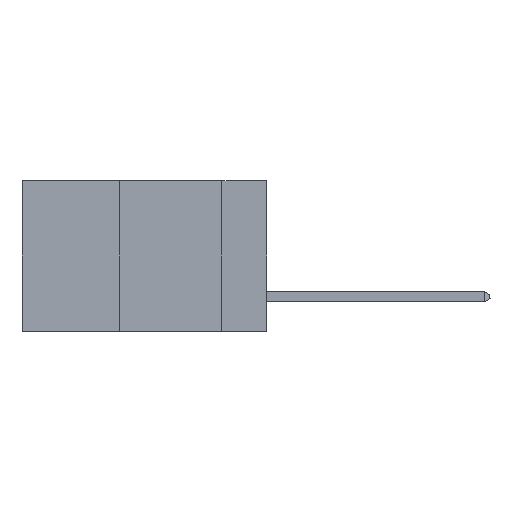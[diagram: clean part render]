
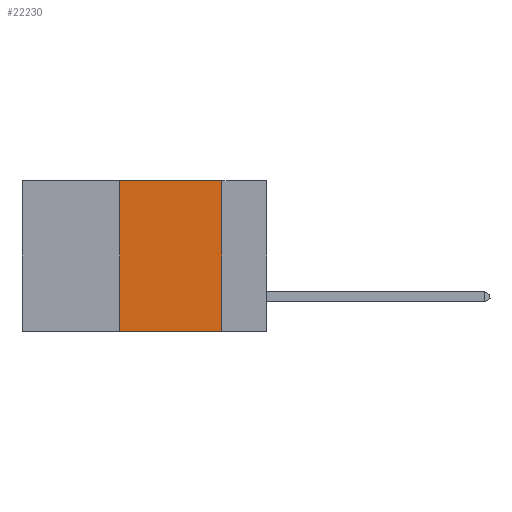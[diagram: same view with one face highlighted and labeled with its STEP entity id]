
A CAD part, left-side view. The second image highlights one B-rep face of the part: STEP entity #22230.
In plain terms, the highlighted planar face has unit normal (-1, 0, 0).
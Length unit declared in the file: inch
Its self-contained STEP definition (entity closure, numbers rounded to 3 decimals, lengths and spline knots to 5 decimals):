
#1137 = FACE_OUTER_BOUND ( 'NONE', #7676, .T. ) ;
#1531 = DIRECTION ( 'NONE',  ( 1., 0., 0. ) ) ;
#2858 = CARTESIAN_POINT ( 'NONE',  ( 0., 0.6, 0. ) ) ;
#3223 = LINE ( 'NONE', #14112, #16207 ) ;
#3950 = EDGE_CURVE ( 'NONE', #8051, #13573, #15029, .T. ) ;
#3980 = CARTESIAN_POINT ( 'NONE',  ( 0., 0.36, -0.37 ) ) ;
#4600 = CARTESIAN_POINT ( 'NONE',  ( 0., 0.36, 0. ) ) ;
#5173 = VERTEX_POINT ( 'NONE', #3980 ) ;
#5322 = PLANE ( 'NONE',  #8281 ) ;
#5871 = DIRECTION ( 'NONE',  ( 0., 0., 1. ) ) ;
#6037 = ORIENTED_EDGE ( 'NONE', *, *, #23399, .F. ) ;
#7606 = VECTOR ( 'NONE', #9836, 39.37008 ) ;
#7676 = EDGE_LOOP ( 'NONE', ( #10054, #6037, #20532, #24123 ) ) ;
#8051 = VERTEX_POINT ( 'NONE', #23278 ) ;
#8281 = AXIS2_PLACEMENT_3D ( 'NONE', #19172, #1531, #17029 ) ;
#9576 = LINE ( 'NONE', #4600, #15479 ) ;
#9676 = CARTESIAN_POINT ( 'NONE',  ( 0., 0.11, -0.37 ) ) ;
#9836 = DIRECTION ( 'NONE',  ( 0., 0., -1. ) ) ;
#10054 = ORIENTED_EDGE ( 'NONE', *, *, #3950, .F. ) ;
#13573 = VERTEX_POINT ( 'NONE', #9676 ) ;
#13943 = DIRECTION ( 'NONE',  ( 0., -1., 0. ) ) ;
#14112 = CARTESIAN_POINT ( 'NONE',  ( 0., 0.6, -0.37 ) ) ;
#14688 = VECTOR ( 'NONE', #18432, 39.37008 ) ;
#15029 = LINE ( 'NONE', #15888, #7606 ) ;
#15479 = VECTOR ( 'NONE', #5871, 39.37008 ) ;
#15656 = EDGE_CURVE ( 'NONE', #5173, #13573, #3223, .T. ) ;
#15888 = CARTESIAN_POINT ( 'NONE',  ( 0., 0.11, 0. ) ) ;
#16207 = VECTOR ( 'NONE', #13943, 39.37008 ) ;
#17029 = DIRECTION ( 'NONE',  ( 0., 0., -1. ) ) ;
#18432 = DIRECTION ( 'NONE',  ( 0., -1., 0. ) ) ;
#19172 = CARTESIAN_POINT ( 'NONE',  ( 0., 0.6, 0. ) ) ;
#19821 = EDGE_CURVE ( 'NONE', #5173, #23567, #9576, .T. ) ;
#20532 = ORIENTED_EDGE ( 'NONE', *, *, #19821, .F. ) ;
#21196 = LINE ( 'NONE', #2858, #14688 ) ;
#22230 = ADVANCED_FACE ( 'NONE', ( #1137 ), #5322, .F. ) ;
#23278 = CARTESIAN_POINT ( 'NONE',  ( 0., 0.11, 0. ) ) ;
#23399 = EDGE_CURVE ( 'NONE', #23567, #8051, #21196, .T. ) ;
#23567 = VERTEX_POINT ( 'NONE', #25288 ) ;
#24123 = ORIENTED_EDGE ( 'NONE', *, *, #15656, .T. ) ;
#25288 = CARTESIAN_POINT ( 'NONE',  ( 0., 0.36, 0. ) ) ;
